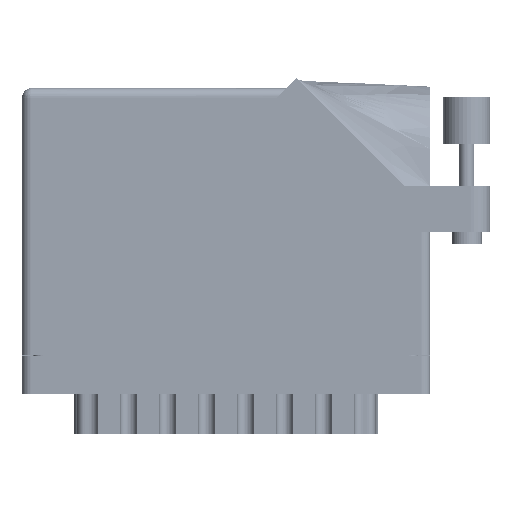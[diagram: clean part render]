
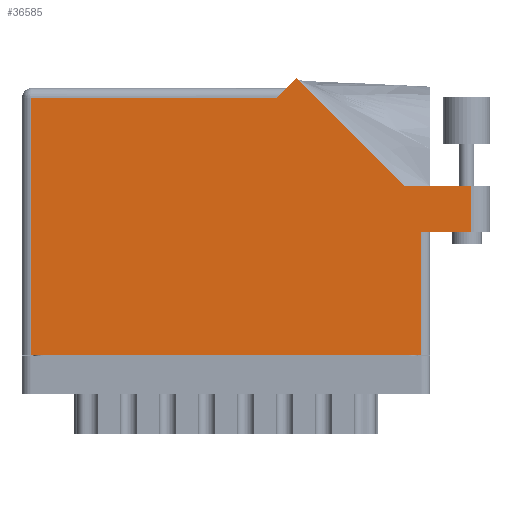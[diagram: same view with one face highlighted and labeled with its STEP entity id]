
A CAD part, front view. The second image highlights one B-rep face of the part: STEP entity #36585.
In plain terms, the highlighted face is planar.
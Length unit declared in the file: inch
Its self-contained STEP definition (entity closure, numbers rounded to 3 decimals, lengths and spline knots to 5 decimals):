
#553 = VECTOR ( 'NONE', #21656, 39.37008 ) ;
#2534 = ORIENTED_EDGE ( 'NONE', *, *, #54177, .T. ) ;
#2536 = ORIENTED_EDGE ( 'NONE', *, *, #5138, .T. ) ;
#3672 = VERTEX_POINT ( 'NONE', #30396 ) ;
#4175 = CARTESIAN_POINT ( 'NONE',  ( 0., 1.713, 0. ) ) ;
#4261 = DIRECTION ( 'NONE',  ( 0., 1., 0. ) ) ;
#4439 = CARTESIAN_POINT ( 'NONE',  ( 2.656, 0.815, 0. ) ) ;
#4682 = CARTESIAN_POINT ( 'NONE',  ( 1.758, 1.775, 0. ) ) ;
#5138 = EDGE_CURVE ( 'NONE', #10033, #3672, #69457, .T. ) ;
#9444 = EDGE_CURVE ( 'NONE', #72352, #59636, #72136, .T. ) ;
#10033 = VERTEX_POINT ( 'NONE', #18162 ) ;
#10331 = DIRECTION ( 'NONE',  ( -0.707, -0.707, 0. ) ) ;
#10524 = EDGE_CURVE ( 'NONE', #48575, #58223, #42941, .T. ) ;
#11274 = ORIENTED_EDGE ( 'NONE', *, *, #27024, .T. ) ;
#11582 = CARTESIAN_POINT ( 'NONE',  ( 0.062, 0., 0. ) ) ;
#12972 = VECTOR ( 'NONE', #72867, 39.37008 ) ;
#13105 = DIRECTION ( 'NONE',  ( 0., 0., -1. ) ) ;
#16337 = CARTESIAN_POINT ( 'NONE',  ( 2.718, 0.815, 0. ) ) ;
#18162 = CARTESIAN_POINT ( 'NONE',  ( 2.656, 0., 0. ) ) ;
#18517 = CARTESIAN_POINT ( 'NONE',  ( 0., 1.775, 0. ) ) ;
#19530 = FACE_OUTER_BOUND ( 'NONE', #26648, .T. ) ;
#20054 = CARTESIAN_POINT ( 'NONE',  ( 2.993, 0.815, 0. ) ) ;
#20434 = CARTESIAN_POINT ( 'NONE',  ( 0.062, 1.713, 0. ) ) ;
#21656 = DIRECTION ( 'NONE',  ( -1., 0., 0. ) ) ;
#21936 = EDGE_CURVE ( 'NONE', #3672, #59796, #27988, .T. ) ;
#22674 = DIRECTION ( 'NONE',  ( 0., -1., 0. ) ) ;
#24057 = EDGE_CURVE ( 'NONE', #59636, #48575, #62116, .T. ) ;
#26648 = EDGE_LOOP ( 'NONE', ( #54576, #2534, #11274, #63939, #40334, #38280, #31092, #32508, #2536 ) ) ;
#27024 = EDGE_CURVE ( 'NONE', #45310, #72352, #34967, .T. ) ;
#27988 = LINE ( 'NONE', #16337, #12972 ) ;
#29733 = VECTOR ( 'NONE', #66447, 39.37008 ) ;
#30396 = CARTESIAN_POINT ( 'NONE',  ( 2.656, 0.815, 0. ) ) ;
#30441 = LINE ( 'NONE', #55540, #52579 ) ;
#31092 = ORIENTED_EDGE ( 'NONE', *, *, #51553, .T. ) ;
#32508 = ORIENTED_EDGE ( 'NONE', *, *, #72864, .T. ) ;
#34723 = VECTOR ( 'NONE', #10331, 39.37008 ) ;
#34967 = LINE ( 'NONE', #70955, #65906 ) ;
#35791 = DIRECTION ( 'NONE',  ( 1., 0., 0. ) ) ;
#36156 = LINE ( 'NONE', #44722, #68003 ) ;
#36585 = ADVANCED_FACE ( 'NONE', ( #19530 ), #46955, .F. ) ;
#37133 = DIRECTION ( 'NONE',  ( -1., 0., 0. ) ) ;
#37349 = CARTESIAN_POINT ( 'NONE',  ( 2.55242, 1.122, 0. ) ) ;
#37620 = AXIS2_PLACEMENT_3D ( 'NONE', #18517, #13105, #64024 ) ;
#38280 = ORIENTED_EDGE ( 'NONE', *, *, #10524, .T. ) ;
#39450 = VECTOR ( 'NONE', #55280, 39.37008 ) ;
#40334 = ORIENTED_EDGE ( 'NONE', *, *, #24057, .T. ) ;
#42941 = LINE ( 'NONE', #4175, #553 ) ;
#43543 = LINE ( 'NONE', #47439, #69165 ) ;
#44722 = CARTESIAN_POINT ( 'NONE',  ( 2.993, 1.122, 0. ) ) ;
#45310 = VERTEX_POINT ( 'NONE', #60599 ) ;
#46935 = CARTESIAN_POINT ( 'NONE',  ( 1.696, 1.713, 0. ) ) ;
#46955 = PLANE ( 'NONE',  #37620 ) ;
#47439 = CARTESIAN_POINT ( 'NONE',  ( 0., 0., 0. ) ) ;
#48575 = VERTEX_POINT ( 'NONE', #46935 ) ;
#51553 = EDGE_CURVE ( 'NONE', #58223, #71477, #30441, .T. ) ;
#52579 = VECTOR ( 'NONE', #22674, 39.37008 ) ;
#54177 = EDGE_CURVE ( 'NONE', #59796, #45310, #36156, .T. ) ;
#54576 = ORIENTED_EDGE ( 'NONE', *, *, #21936, .T. ) ;
#55280 = DIRECTION ( 'NONE',  ( 0., 1., 0. ) ) ;
#55540 = CARTESIAN_POINT ( 'NONE',  ( 0.062, 0., 0. ) ) ;
#58223 = VERTEX_POINT ( 'NONE', #20434 ) ;
#59636 = VERTEX_POINT ( 'NONE', #70387 ) ;
#59796 = VERTEX_POINT ( 'NONE', #20054 ) ;
#60599 = CARTESIAN_POINT ( 'NONE',  ( 2.993, 1.122, 0. ) ) ;
#62116 = LINE ( 'NONE', #4682, #34723 ) ;
#63939 = ORIENTED_EDGE ( 'NONE', *, *, #9444, .T. ) ;
#64024 = DIRECTION ( 'NONE',  ( -1., 0., 0. ) ) ;
#65906 = VECTOR ( 'NONE', #37133, 39.37008 ) ;
#66447 = DIRECTION ( 'NONE',  ( -0.707, 0.707, 0. ) ) ;
#66689 = CARTESIAN_POINT ( 'NONE',  ( 2.55242, 1.122, 0. ) ) ;
#68003 = VECTOR ( 'NONE', #4261, 39.37008 ) ;
#69165 = VECTOR ( 'NONE', #35791, 39.37008 ) ;
#69457 = LINE ( 'NONE', #4439, #39450 ) ;
#70387 = CARTESIAN_POINT ( 'NONE',  ( 1.82871, 1.84571, 0. ) ) ;
#70955 = CARTESIAN_POINT ( 'NONE',  ( 3.118, 1.122, 0. ) ) ;
#71477 = VERTEX_POINT ( 'NONE', #11582 ) ;
#72136 = LINE ( 'NONE', #66689, #29733 ) ;
#72352 = VERTEX_POINT ( 'NONE', #37349 ) ;
#72864 = EDGE_CURVE ( 'NONE', #71477, #10033, #43543, .T. ) ;
#72867 = DIRECTION ( 'NONE',  ( 1., 0., 0. ) ) ;
